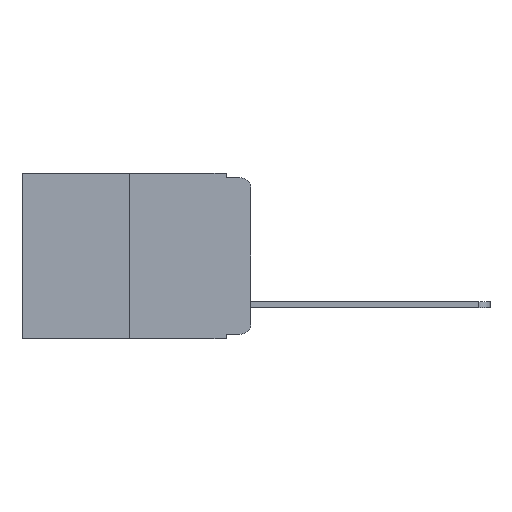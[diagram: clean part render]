
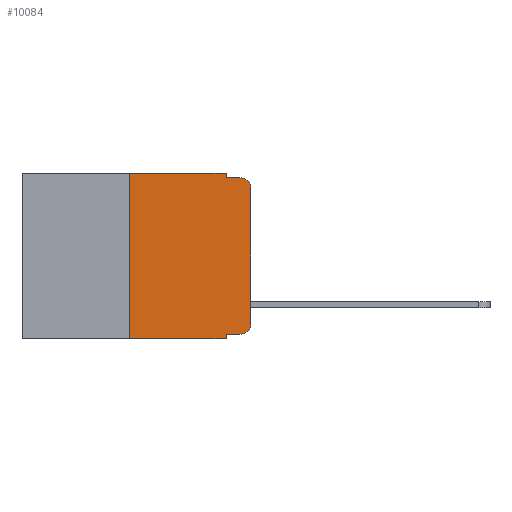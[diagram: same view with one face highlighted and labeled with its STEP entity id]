
A CAD part, left-side view. The second image highlights one B-rep face of the part: STEP entity #10084.
In plain terms, the highlighted planar face has unit normal (-1, 0, 0).
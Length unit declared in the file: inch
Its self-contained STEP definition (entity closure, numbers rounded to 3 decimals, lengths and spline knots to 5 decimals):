
#280 = CARTESIAN_POINT ( 'NONE',  ( 0., 0.051, -0.343 ) ) ;
#345 = DIRECTION ( 'NONE',  ( 0., 0., -1. ) ) ;
#710 = DIRECTION ( 'NONE',  ( 0., -1., 0. ) ) ;
#1083 = VERTEX_POINT ( 'NONE', #9744 ) ;
#1360 = DIRECTION ( 'NONE',  ( 0., 0., -1. ) ) ;
#2212 = CARTESIAN_POINT ( 'NONE',  ( 0., 0.02, -0.313 ) ) ;
#2274 = VERTEX_POINT ( 'NONE', #11947 ) ;
#2806 = LINE ( 'NONE', #19294, #11336 ) ;
#2976 = CARTESIAN_POINT ( 'NONE',  ( 0., 0.02, -0.03 ) ) ;
#3033 = CARTESIAN_POINT ( 'NONE',  ( 0., 0.25, 0. ) ) ;
#3144 = AXIS2_PLACEMENT_3D ( 'NONE', #2212, #3788, #345 ) ;
#3192 = ORIENTED_EDGE ( 'NONE', *, *, #14728, .T. ) ;
#3210 = VECTOR ( 'NONE', #710, 39.37008 ) ;
#3366 = ORIENTED_EDGE ( 'NONE', *, *, #10919, .T. ) ;
#3788 = DIRECTION ( 'NONE',  ( -1., 0., 0. ) ) ;
#3885 = LINE ( 'NONE', #14641, #18821 ) ;
#4185 = ORIENTED_EDGE ( 'NONE', *, *, #16262, .T. ) ;
#4480 = AXIS2_PLACEMENT_3D ( 'NONE', #11305, #12737, #9491 ) ;
#4879 = CARTESIAN_POINT ( 'NONE',  ( 0., 0.051, 0. ) ) ;
#5152 = EDGE_CURVE ( 'NONE', #10272, #8943, #13911, .T. ) ;
#5242 = VECTOR ( 'NONE', #5925, 39.37008 ) ;
#5925 = DIRECTION ( 'NONE',  ( 0., 0., 1. ) ) ;
#6279 = DIRECTION ( 'NONE',  ( -1., 0., 0. ) ) ;
#6636 = DIRECTION ( 'NONE',  ( 0., -1., 0. ) ) ;
#7233 = CARTESIAN_POINT ( 'NONE',  ( 0., 0.051, -0.01 ) ) ;
#7580 = ORIENTED_EDGE ( 'NONE', *, *, #10368, .F. ) ;
#7634 = CIRCLE ( 'NONE', #3144, 0.02 ) ;
#7872 = LINE ( 'NONE', #11589, #14547 ) ;
#8840 = CIRCLE ( 'NONE', #13035, 0.02 ) ;
#8921 = CARTESIAN_POINT ( 'NONE',  ( 0., 0.473, 0. ) ) ;
#8943 = VERTEX_POINT ( 'NONE', #16075 ) ;
#9189 = ORIENTED_EDGE ( 'NONE', *, *, #16610, .F. ) ;
#9491 = DIRECTION ( 'NONE',  ( 0., 0., -1. ) ) ;
#9744 = CARTESIAN_POINT ( 'NONE',  ( 0., 0.25, 0. ) ) ;
#10072 = VERTEX_POINT ( 'NONE', #4879 ) ;
#10084 = ADVANCED_FACE ( 'NONE', ( #10152 ), #21116, .F. ) ;
#10147 = VERTEX_POINT ( 'NONE', #11173 ) ;
#10152 = FACE_OUTER_BOUND ( 'NONE', #16526, .T. ) ;
#10272 = VERTEX_POINT ( 'NONE', #14657 ) ;
#10368 = EDGE_CURVE ( 'NONE', #12456, #1083, #10651, .T. ) ;
#10651 = LINE ( 'NONE', #3033, #5242 ) ;
#10919 = EDGE_CURVE ( 'NONE', #10147, #2274, #8840, .T. ) ;
#11016 = EDGE_CURVE ( 'NONE', #14232, #2274, #18588, .T. ) ;
#11129 = CARTESIAN_POINT ( 'NONE',  ( 0., 0., -0.313 ) ) ;
#11173 = CARTESIAN_POINT ( 'NONE',  ( 0., 0., -0.03 ) ) ;
#11294 = DIRECTION ( 'NONE',  ( 0., 0., 1. ) ) ;
#11305 = CARTESIAN_POINT ( 'NONE',  ( 0., 0.473, 0. ) ) ;
#11336 = VECTOR ( 'NONE', #1360, 39.37008 ) ;
#11564 = CARTESIAN_POINT ( 'NONE',  ( 0., 0.051, -0.333 ) ) ;
#11589 = CARTESIAN_POINT ( 'NONE',  ( 0., 0.473, -0.343 ) ) ;
#11592 = ORIENTED_EDGE ( 'NONE', *, *, #5152, .T. ) ;
#11947 = CARTESIAN_POINT ( 'NONE',  ( 0., 0.02, -0.01 ) ) ;
#12203 = DIRECTION ( 'NONE',  ( 0., -1., 0. ) ) ;
#12456 = VERTEX_POINT ( 'NONE', #13103 ) ;
#12737 = DIRECTION ( 'NONE',  ( 1., 0., 0. ) ) ;
#12898 = LINE ( 'NONE', #13151, #19320 ) ;
#13035 = AXIS2_PLACEMENT_3D ( 'NONE', #2976, #6279, #17794 ) ;
#13103 = CARTESIAN_POINT ( 'NONE',  ( 0., 0.25, -0.343 ) ) ;
#13151 = CARTESIAN_POINT ( 'NONE',  ( 0., 0., 0. ) ) ;
#13508 = VERTEX_POINT ( 'NONE', #11129 ) ;
#13821 = CARTESIAN_POINT ( 'NONE',  ( 0., 0.051, -0.01 ) ) ;
#13911 = LINE ( 'NONE', #11564, #20834 ) ;
#14232 = VERTEX_POINT ( 'NONE', #13821 ) ;
#14547 = VECTOR ( 'NONE', #16024, 39.37008 ) ;
#14641 = CARTESIAN_POINT ( 'NONE',  ( 0., 0.051, 0. ) ) ;
#14657 = CARTESIAN_POINT ( 'NONE',  ( 0., 0.051, -0.333 ) ) ;
#14728 = EDGE_CURVE ( 'NONE', #8943, #13508, #7634, .T. ) ;
#14799 = LINE ( 'NONE', #8921, #3210 ) ;
#15485 = VECTOR ( 'NONE', #12203, 39.37008 ) ;
#16024 = DIRECTION ( 'NONE',  ( 0., -1., 0. ) ) ;
#16075 = CARTESIAN_POINT ( 'NONE',  ( 0., 0.02, -0.333 ) ) ;
#16221 = ORIENTED_EDGE ( 'NONE', *, *, #19743, .F. ) ;
#16262 = EDGE_CURVE ( 'NONE', #12456, #16869, #7872, .T. ) ;
#16526 = EDGE_LOOP ( 'NONE', ( #19540, #3366, #16996, #16221, #9189, #7580, #4185, #18539, #11592, #3192 ) ) ;
#16610 = EDGE_CURVE ( 'NONE', #1083, #10072, #14799, .T. ) ;
#16869 = VERTEX_POINT ( 'NONE', #280 ) ;
#16996 = ORIENTED_EDGE ( 'NONE', *, *, #11016, .F. ) ;
#17794 = DIRECTION ( 'NONE',  ( 0., 0., -1. ) ) ;
#18539 = ORIENTED_EDGE ( 'NONE', *, *, #19170, .F. ) ;
#18588 = LINE ( 'NONE', #7233, #15485 ) ;
#18821 = VECTOR ( 'NONE', #19610, 39.37008 ) ;
#19170 = EDGE_CURVE ( 'NONE', #10272, #16869, #3885, .T. ) ;
#19262 = EDGE_CURVE ( 'NONE', #13508, #10147, #12898, .T. ) ;
#19294 = CARTESIAN_POINT ( 'NONE',  ( 0., 0.051, 0. ) ) ;
#19320 = VECTOR ( 'NONE', #11294, 39.37008 ) ;
#19540 = ORIENTED_EDGE ( 'NONE', *, *, #19262, .T. ) ;
#19610 = DIRECTION ( 'NONE',  ( 0., 0., -1. ) ) ;
#19743 = EDGE_CURVE ( 'NONE', #10072, #14232, #2806, .T. ) ;
#20834 = VECTOR ( 'NONE', #6636, 39.37008 ) ;
#21116 = PLANE ( 'NONE',  #4480 ) ;
